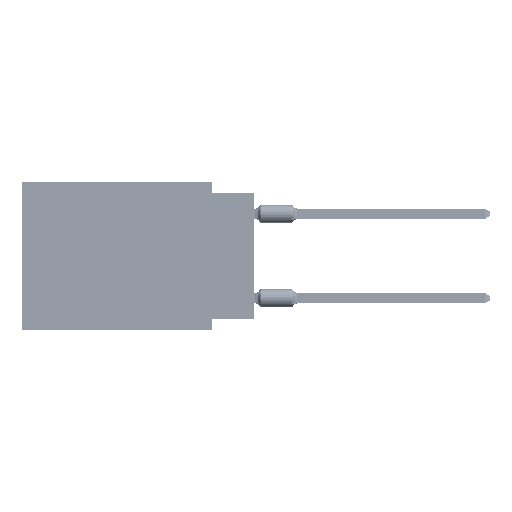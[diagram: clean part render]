
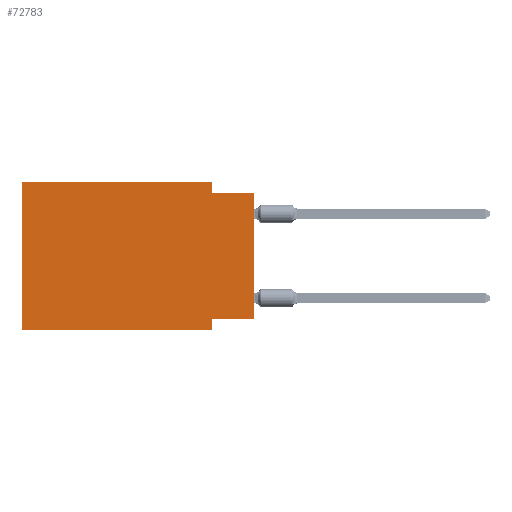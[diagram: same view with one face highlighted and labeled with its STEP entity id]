
A CAD part, left-side view. The second image highlights one B-rep face of the part: STEP entity #72783.
In plain terms, the highlighted planar face has unit normal (-1, 0, 0).
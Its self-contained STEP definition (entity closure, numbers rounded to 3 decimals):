
#1384 = EDGE_CURVE ( 'NONE', #3293, #83961, #25481, .T. ) ;
#2429 = EDGE_CURVE ( 'NONE', #66821, #70131, #79336, .T. ) ;
#2649 = DIRECTION ( 'NONE',  ( 0., 0., -1. ) ) ;
#3293 = VERTEX_POINT ( 'NONE', #43219 ) ;
#7254 = CARTESIAN_POINT ( 'NONE',  ( 0., 0., -0.635 ) ) ;
#8310 = LINE ( 'NONE', #22532, #12250 ) ;
#9040 = ORIENTED_EDGE ( 'NONE', *, *, #56753, .F. ) ;
#10216 = EDGE_CURVE ( 'NONE', #29924, #77381, #34854, .T. ) ;
#10686 = ORIENTED_EDGE ( 'NONE', *, *, #39401, .F. ) ;
#11701 = CARTESIAN_POINT ( 'NONE',  ( 0., 13.97, 0. ) ) ;
#11995 = CARTESIAN_POINT ( 'NONE',  ( 0., 2.54, 0. ) ) ;
#12250 = VECTOR ( 'NONE', #64325, 1000. ) ;
#12682 = CARTESIAN_POINT ( 'NONE',  ( 0., 0., -8.255 ) ) ;
#12915 = CARTESIAN_POINT ( 'NONE',  ( 0., 2.54, -8.89 ) ) ;
#14028 = CARTESIAN_POINT ( 'NONE',  ( 0., 2.54, -8.89 ) ) ;
#21059 = DIRECTION ( 'NONE',  ( 0., 0., 1. ) ) ;
#21617 = LINE ( 'NONE', #85412, #41209 ) ;
#22532 = CARTESIAN_POINT ( 'NONE',  ( 0., 13.97, 0. ) ) ;
#23314 = EDGE_LOOP ( 'NONE', ( #60414, #10686, #76989, #83905, #34559, #84367, #35892, #9040 ) ) ;
#24716 = EDGE_CURVE ( 'NONE', #87326, #55800, #54217, .T. ) ;
#25481 = LINE ( 'NONE', #11701, #67323 ) ;
#25554 = LINE ( 'NONE', #12682, #27354 ) ;
#27354 = VECTOR ( 'NONE', #88923, 1000. ) ;
#29924 = VERTEX_POINT ( 'NONE', #85303 ) ;
#32144 = VECTOR ( 'NONE', #48258, 1000. ) ;
#34559 = ORIENTED_EDGE ( 'NONE', *, *, #1384, .F. ) ;
#34854 = LINE ( 'NONE', #62842, #62573 ) ;
#35892 = ORIENTED_EDGE ( 'NONE', *, *, #24716, .F. ) ;
#38088 = VECTOR ( 'NONE', #2649, 1000. ) ;
#38197 = LINE ( 'NONE', #38638, #79477 ) ;
#38331 = EDGE_CURVE ( 'NONE', #3293, #55800, #21617, .T. ) ;
#38638 = CARTESIAN_POINT ( 'NONE',  ( 0., 0., -0.635 ) ) ;
#39401 = EDGE_CURVE ( 'NONE', #70131, #77381, #38197, .T. ) ;
#39706 = DIRECTION ( 'NONE',  ( 0., 0., 1. ) ) ;
#41209 = VECTOR ( 'NONE', #69823, 1000. ) ;
#42041 = AXIS2_PLACEMENT_3D ( 'NONE', #49999, #42673, #78457 ) ;
#42320 = CARTESIAN_POINT ( 'NONE',  ( 0., 13.97, 0. ) ) ;
#42673 = DIRECTION ( 'NONE',  ( 1., 0., 0. ) ) ;
#43114 = FACE_OUTER_BOUND ( 'NONE', #23314, .T. ) ;
#43219 = CARTESIAN_POINT ( 'NONE',  ( 0., 13.97, -8.89 ) ) ;
#44422 = CARTESIAN_POINT ( 'NONE',  ( 0., 2.54, 0. ) ) ;
#48258 = DIRECTION ( 'NONE',  ( 0., 0., -1. ) ) ;
#49999 = CARTESIAN_POINT ( 'NONE',  ( 0., 13.97, 0. ) ) ;
#52292 = CARTESIAN_POINT ( 'NONE',  ( 0., 2.54, -8.255 ) ) ;
#54217 = LINE ( 'NONE', #12915, #32144 ) ;
#55800 = VERTEX_POINT ( 'NONE', #14028 ) ;
#56753 = EDGE_CURVE ( 'NONE', #29924, #87326, #25554, .T. ) ;
#58576 = CARTESIAN_POINT ( 'NONE',  ( 0., 2.54, -0.635 ) ) ;
#60414 = ORIENTED_EDGE ( 'NONE', *, *, #10216, .T. ) ;
#62573 = VECTOR ( 'NONE', #21059, 1000. ) ;
#62842 = CARTESIAN_POINT ( 'NONE',  ( 0., 0., 0. ) ) ;
#64325 = DIRECTION ( 'NONE',  ( 0., -1., 0. ) ) ;
#66821 = VERTEX_POINT ( 'NONE', #11995 ) ;
#67323 = VECTOR ( 'NONE', #39706, 1000. ) ;
#69823 = DIRECTION ( 'NONE',  ( 0., -1., 0. ) ) ;
#70131 = VERTEX_POINT ( 'NONE', #58576 ) ;
#72783 = ADVANCED_FACE ( 'NONE', ( #43114 ), #86273, .F. ) ;
#76989 = ORIENTED_EDGE ( 'NONE', *, *, #2429, .F. ) ;
#77381 = VERTEX_POINT ( 'NONE', #7254 ) ;
#78457 = DIRECTION ( 'NONE',  ( 0., 0., -1. ) ) ;
#79336 = LINE ( 'NONE', #44422, #38088 ) ;
#79477 = VECTOR ( 'NONE', #87344, 1000. ) ;
#81157 = EDGE_CURVE ( 'NONE', #83961, #66821, #8310, .T. ) ;
#83905 = ORIENTED_EDGE ( 'NONE', *, *, #81157, .F. ) ;
#83961 = VERTEX_POINT ( 'NONE', #42320 ) ;
#84367 = ORIENTED_EDGE ( 'NONE', *, *, #38331, .T. ) ;
#85303 = CARTESIAN_POINT ( 'NONE',  ( 0., 0., -8.255 ) ) ;
#85412 = CARTESIAN_POINT ( 'NONE',  ( 0., 13.97, -8.89 ) ) ;
#86273 = PLANE ( 'NONE',  #42041 ) ;
#87326 = VERTEX_POINT ( 'NONE', #52292 ) ;
#87344 = DIRECTION ( 'NONE',  ( 0., -1., 0. ) ) ;
#88923 = DIRECTION ( 'NONE',  ( 0., 1., 0. ) ) ;
